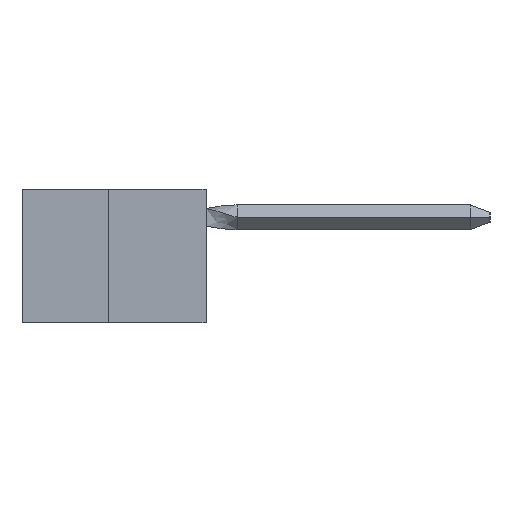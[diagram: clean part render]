
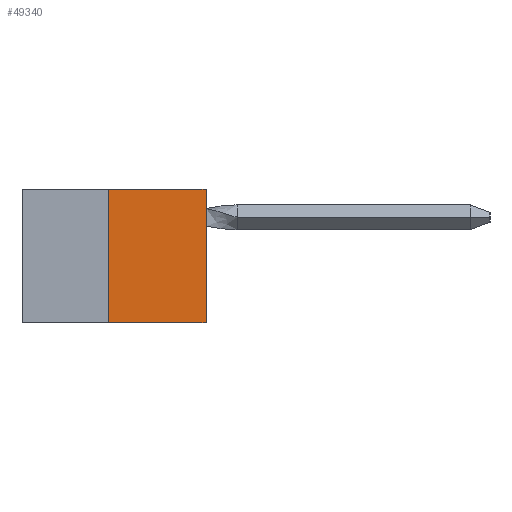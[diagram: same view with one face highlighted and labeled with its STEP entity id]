
A CAD part, left-side view. The second image highlights one B-rep face of the part: STEP entity #49340.
In plain terms, the highlighted planar face has unit normal (-1, 0, 0).
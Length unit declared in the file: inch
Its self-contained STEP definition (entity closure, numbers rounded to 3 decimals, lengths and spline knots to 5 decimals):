
#6518 = ORIENTED_EDGE ( 'NONE', *, *, #45884, .T. ) ;
#7110 = ORIENTED_EDGE ( 'NONE', *, *, #51111, .T. ) ;
#9895 = LINE ( 'NONE', #46508, #44504 ) ;
#12370 = DIRECTION ( 'NONE',  ( 0., 0., 1. ) ) ;
#13145 = EDGE_CURVE ( 'NONE', #26970, #41343, #55536, .T. ) ;
#14087 = PLANE ( 'NONE',  #37828 ) ;
#14328 = EDGE_CURVE ( 'NONE', #49247, #26970, #9895, .T. ) ;
#16853 = ORIENTED_EDGE ( 'NONE', *, *, #13145, .F. ) ;
#19030 = CARTESIAN_POINT ( 'NONE',  ( 0., 0.473, 0. ) ) ;
#21880 = CARTESIAN_POINT ( 'NONE',  ( 0., 0.25, -0.343 ) ) ;
#22765 = DIRECTION ( 'NONE',  ( 0., -1., 0. ) ) ;
#24125 = DIRECTION ( 'NONE',  ( 1., 0., 0. ) ) ;
#26970 = VERTEX_POINT ( 'NONE', #37544 ) ;
#28764 = CARTESIAN_POINT ( 'NONE',  ( 0., 0., 0. ) ) ;
#30176 = VERTEX_POINT ( 'NONE', #54236 ) ;
#33125 = VECTOR ( 'NONE', #47315, 39.37008 ) ;
#35476 = DIRECTION ( 'NONE',  ( 0., 0., -1. ) ) ;
#37544 = CARTESIAN_POINT ( 'NONE',  ( 0., 0.25, 0. ) ) ;
#37828 = AXIS2_PLACEMENT_3D ( 'NONE', #19030, #24125, #35476 ) ;
#38922 = CARTESIAN_POINT ( 'NONE',  ( 0., 0.473, 0. ) ) ;
#39430 = DIRECTION ( 'NONE',  ( 0., 0., 1. ) ) ;
#40340 = ORIENTED_EDGE ( 'NONE', *, *, #14328, .F. ) ;
#40439 = FACE_OUTER_BOUND ( 'NONE', #47995, .T. ) ;
#40468 = LINE ( 'NONE', #43448, #47305 ) ;
#41343 = VERTEX_POINT ( 'NONE', #28764 ) ;
#42122 = LINE ( 'NONE', #44757, #46878 ) ;
#43448 = CARTESIAN_POINT ( 'NONE',  ( 0., 0., 0. ) ) ;
#44504 = VECTOR ( 'NONE', #12370, 39.37008 ) ;
#44757 = CARTESIAN_POINT ( 'NONE',  ( 0., 0.473, -0.343 ) ) ;
#45884 = EDGE_CURVE ( 'NONE', #49247, #30176, #42122, .T. ) ;
#46508 = CARTESIAN_POINT ( 'NONE',  ( 0., 0.25, 0. ) ) ;
#46878 = VECTOR ( 'NONE', #22765, 39.37008 ) ;
#47305 = VECTOR ( 'NONE', #39430, 39.37008 ) ;
#47315 = DIRECTION ( 'NONE',  ( 0., -1., 0. ) ) ;
#47995 = EDGE_LOOP ( 'NONE', ( #16853, #40340, #6518, #7110 ) ) ;
#49247 = VERTEX_POINT ( 'NONE', #21880 ) ;
#49340 = ADVANCED_FACE ( 'NONE', ( #40439 ), #14087, .F. ) ;
#51111 = EDGE_CURVE ( 'NONE', #30176, #41343, #40468, .T. ) ;
#54236 = CARTESIAN_POINT ( 'NONE',  ( 0., 0., -0.343 ) ) ;
#55536 = LINE ( 'NONE', #38922, #33125 ) ;
